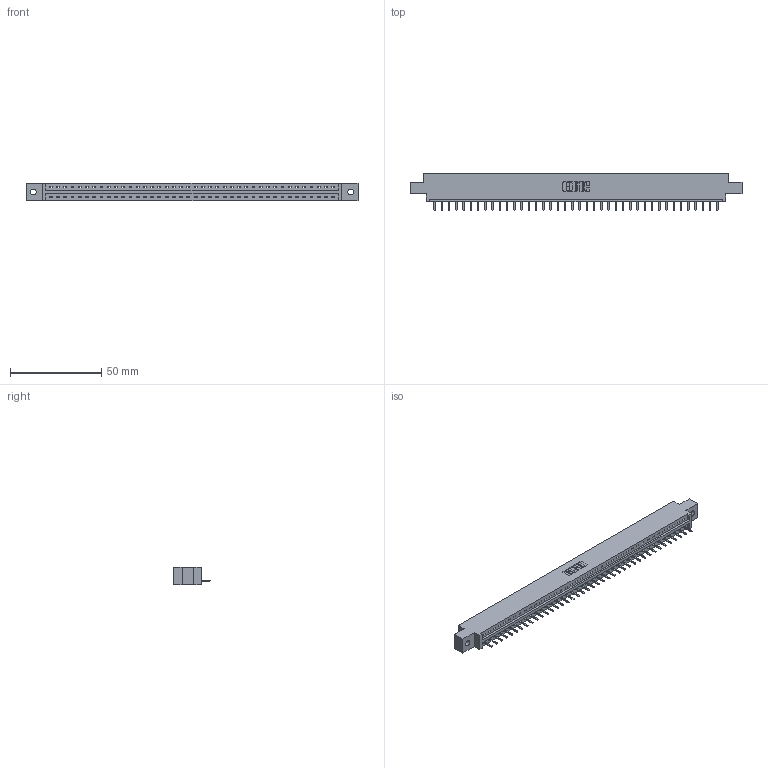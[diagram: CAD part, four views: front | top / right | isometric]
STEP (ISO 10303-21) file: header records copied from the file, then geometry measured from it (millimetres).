
FILE_DESCRIPTION (( 'STEP AP203' ), '1' );
FILE_NAME ('387-040-520-602.STEP', '2018-09-19T09:27:51', ( '' ), ( '' ), 'SwSTEP 2.0', 'SolidWorks 2016', '' );
FILE_SCHEMA (( 'CONFIG_CONTROL_DESIGN' ));
Length unit declared in the file: inch
Products named in the file (3): 337 Part_0.170 Offset - 0.128 Dia; 345-292-001_345-293-120; 387-040-520-602
Assembly tree (41 placements, depth 2):
  387-040-520-602
    337 Part_0.170 Offset - 0.128 Dia
    345-292-001_345-293-120  x40
Bounding box: 181.51 x 20.02 x 9.4 mm (x, y, z)
Volume: 18570.5 mm3; surface area: 18591.1 mm2
Topology: 41 solids, 41 shells, 2758 faces, 8163 edges, 5334 vertices
Faces by surface type: plane 1994, cylinder 764
Entity records: 30241 total; most frequent: CARTESIAN_POINT 5286, ORIENTED_EDGE 5250, DIRECTION 4441, EDGE_CURVE 2625, VECTOR 2493, LINE 2493, VERTEX_POINT 1746, AXIS2_PLACEMENT_3D 974
